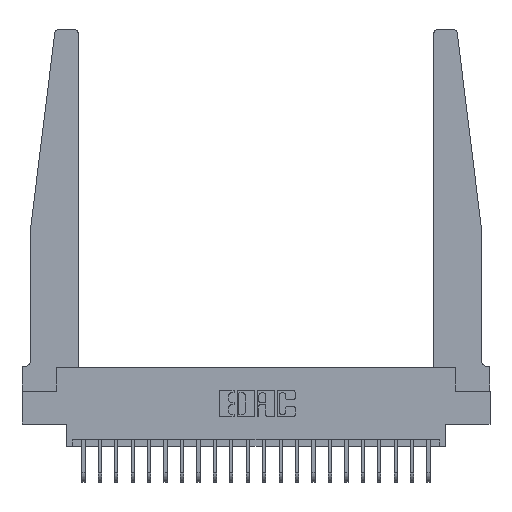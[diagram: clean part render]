
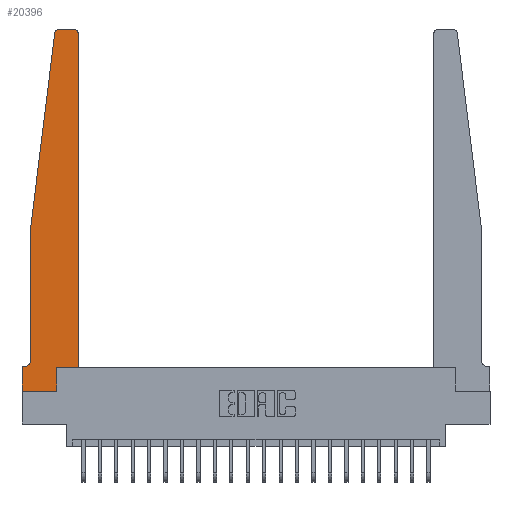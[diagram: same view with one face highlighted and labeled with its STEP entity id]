
A CAD part, top view. The second image highlights one B-rep face of the part: STEP entity #20396.
In plain terms, the highlighted planar face has unit normal (0, 0, 1).
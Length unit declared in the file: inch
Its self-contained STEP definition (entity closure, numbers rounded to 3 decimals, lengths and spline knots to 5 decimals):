
#13 = VERTEX_POINT ( 'NONE', #19878 ) ;
#154 = EDGE_CURVE ( 'NONE', #13275, #3862, #9523, .T. ) ;
#205 = VERTEX_POINT ( 'NONE', #922 ) ;
#274 = FACE_OUTER_BOUND ( 'NONE', #7038, .T. ) ;
#571 = CARTESIAN_POINT ( 'NONE',  ( 0., 0.1875, 0.37 ) ) ;
#922 = CARTESIAN_POINT ( 'NONE',  ( 0., 0., 0.37 ) ) ;
#1154 = EDGE_CURVE ( 'NONE', #13, #10740, #17629, .T. ) ;
#1171 = VECTOR ( 'NONE', #15582, 39.37008 ) ;
#1289 = CARTESIAN_POINT ( 'NONE',  ( 0., 0.1875, 0.37 ) ) ;
#2060 = VERTEX_POINT ( 'NONE', #20633 ) ;
#2206 = DIRECTION ( 'NONE',  ( 0., -1., 0. ) ) ;
#2225 = EDGE_CURVE ( 'NONE', #18120, #14885, #20172, .T. ) ;
#2480 = CARTESIAN_POINT ( 'NONE',  ( 0.2605, 0.18, 0.37 ) ) ;
#2614 = VECTOR ( 'NONE', #15246, 39.37008 ) ;
#2959 = DIRECTION ( 'NONE',  ( 1., 0., 0. ) ) ;
#3047 = LINE ( 'NONE', #4867, #7074 ) ;
#3566 = AXIS2_PLACEMENT_3D ( 'NONE', #14869, #5004, #16492 ) ;
#3673 = CARTESIAN_POINT ( 'NONE',  ( 0.395, 2.72, 0.37 ) ) ;
#3862 = VERTEX_POINT ( 'NONE', #5799 ) ;
#4046 = CIRCLE ( 'NONE', #3566, 0.03 ) ;
#4161 = CARTESIAN_POINT ( 'NONE',  ( 0.065, 1.25, 0.37 ) ) ;
#4199 = CARTESIAN_POINT ( 'NONE',  ( 0.425, 0.18, 0.37 ) ) ;
#4451 = ORIENTED_EDGE ( 'NONE', *, *, #12958, .T. ) ;
#4606 = CIRCLE ( 'NONE', #12302, 0.05 ) ;
#4867 = CARTESIAN_POINT ( 'NONE',  ( 0.425, 0.18, 0.37 ) ) ;
#4990 = ORIENTED_EDGE ( 'NONE', *, *, #1154, .T. ) ;
#5004 = DIRECTION ( 'NONE',  ( 0., 0., 1. ) ) ;
#5237 = ORIENTED_EDGE ( 'NONE', *, *, #8057, .T. ) ;
#5434 = DIRECTION ( 'NONE',  ( 1., 0., 0. ) ) ;
#5516 = ORIENTED_EDGE ( 'NONE', *, *, #20247, .T. ) ;
#5532 = EDGE_CURVE ( 'NONE', #12463, #2060, #11988, .T. ) ;
#5782 = CARTESIAN_POINT ( 'NONE',  ( 0., 0., 0.37 ) ) ;
#5799 = CARTESIAN_POINT ( 'NONE',  ( 0.065, 1.25, 0.37 ) ) ;
#6256 = VECTOR ( 'NONE', #2206, 39.37008 ) ;
#6421 = EDGE_CURVE ( 'NONE', #2060, #12313, #3047, .T. ) ;
#6766 = DIRECTION ( 'NONE',  ( 0., 0., -1. ) ) ;
#6806 = CARTESIAN_POINT ( 'NONE',  ( 0.25, 2.75, 0.37 ) ) ;
#7019 = CARTESIAN_POINT ( 'NONE',  ( 0.065, 0.1875, 0.37 ) ) ;
#7038 = EDGE_LOOP ( 'NONE', ( #4990, #4451, #19062, #10424, #18548, #14259, #5516, #13218, #8338, #16521, #14012, #5237 ) ) ;
#7074 = VECTOR ( 'NONE', #17970, 39.37008 ) ;
#7398 = VECTOR ( 'NONE', #10972, 39.37008 ) ;
#7460 = EDGE_CURVE ( 'NONE', #3862, #13134, #19252, .T. ) ;
#7509 = EDGE_CURVE ( 'NONE', #205, #12463, #18748, .T. ) ;
#7673 = CARTESIAN_POINT ( 'NONE',  ( 0., 0., 0.37 ) ) ;
#7940 = CARTESIAN_POINT ( 'NONE',  ( 0.27653, 2.75, 0.37 ) ) ;
#8057 = EDGE_CURVE ( 'NONE', #20066, #13, #17496, .T. ) ;
#8255 = CARTESIAN_POINT ( 'NONE',  ( 0.425, 0.18, 0.37 ) ) ;
#8338 = ORIENTED_EDGE ( 'NONE', *, *, #5532, .T. ) ;
#8434 = DIRECTION ( 'NONE',  ( -1., 0., 0. ) ) ;
#8803 = VECTOR ( 'NONE', #13204, 39.37008 ) ;
#9523 = LINE ( 'NONE', #4161, #17178 ) ;
#9659 = PLANE ( 'NONE',  #12207 ) ;
#10424 = ORIENTED_EDGE ( 'NONE', *, *, #7460, .T. ) ;
#10740 = VERTEX_POINT ( 'NONE', #7940 ) ;
#10853 = DIRECTION ( 'NONE',  ( 0., 1., 0. ) ) ;
#10972 = DIRECTION ( 'NONE',  ( 0., -1., 0. ) ) ;
#11455 = EDGE_CURVE ( 'NONE', #12313, #20066, #13160, .T. ) ;
#11749 = LINE ( 'NONE', #7673, #7398 ) ;
#11988 = LINE ( 'NONE', #2480, #19092 ) ;
#12207 = AXIS2_PLACEMENT_3D ( 'NONE', #1289, #12953, #2959 ) ;
#12302 = AXIS2_PLACEMENT_3D ( 'NONE', #16537, #6766, #18155 ) ;
#12313 = VERTEX_POINT ( 'NONE', #4199 ) ;
#12463 = VERTEX_POINT ( 'NONE', #19267 ) ;
#12953 = DIRECTION ( 'NONE',  ( 0., 0., 1. ) ) ;
#12958 = EDGE_CURVE ( 'NONE', #10740, #13275, #4046, .T. ) ;
#13134 = VERTEX_POINT ( 'NONE', #16837 ) ;
#13160 = LINE ( 'NONE', #8255, #8803 ) ;
#13204 = DIRECTION ( 'NONE',  ( 0., 1., 0. ) ) ;
#13218 = ORIENTED_EDGE ( 'NONE', *, *, #7509, .T. ) ;
#13275 = VERTEX_POINT ( 'NONE', #18811 ) ;
#13870 = CARTESIAN_POINT ( 'NONE',  ( 0.065, 1.25, 0.37 ) ) ;
#14012 = ORIENTED_EDGE ( 'NONE', *, *, #11455, .T. ) ;
#14259 = ORIENTED_EDGE ( 'NONE', *, *, #2225, .T. ) ;
#14869 = CARTESIAN_POINT ( 'NONE',  ( 0.27653, 2.72, 0.37 ) ) ;
#14885 = VERTEX_POINT ( 'NONE', #571 ) ;
#14989 = AXIS2_PLACEMENT_3D ( 'NONE', #3673, #15273, #5434 ) ;
#15246 = DIRECTION ( 'NONE',  ( -1., 0., 0. ) ) ;
#15273 = DIRECTION ( 'NONE',  ( 0., 0., 1. ) ) ;
#15582 = DIRECTION ( 'NONE',  ( 1., 0., 0. ) ) ;
#15711 = DIRECTION ( 'NONE',  ( -0.122, -0.992, 0. ) ) ;
#16492 = DIRECTION ( 'NONE',  ( 1., 0., 0. ) ) ;
#16521 = ORIENTED_EDGE ( 'NONE', *, *, #6421, .T. ) ;
#16537 = CARTESIAN_POINT ( 'NONE',  ( 0.015, 0.2375, 0.37 ) ) ;
#16837 = CARTESIAN_POINT ( 'NONE',  ( 0.065, 0.2375, 0.37 ) ) ;
#17178 = VECTOR ( 'NONE', #15711, 39.37008 ) ;
#17496 = CIRCLE ( 'NONE', #14989, 0.03 ) ;
#17629 = LINE ( 'NONE', #6806, #18644 ) ;
#17731 = EDGE_CURVE ( 'NONE', #13134, #18120, #4606, .T. ) ;
#17970 = DIRECTION ( 'NONE',  ( 1., 0., 0. ) ) ;
#18120 = VERTEX_POINT ( 'NONE', #20639 ) ;
#18155 = DIRECTION ( 'NONE',  ( -1., 0., 0. ) ) ;
#18548 = ORIENTED_EDGE ( 'NONE', *, *, #17731, .T. ) ;
#18644 = VECTOR ( 'NONE', #8434, 39.37008 ) ;
#18748 = LINE ( 'NONE', #5782, #1171 ) ;
#18811 = CARTESIAN_POINT ( 'NONE',  ( 0.24675, 2.72367, 0.37 ) ) ;
#19062 = ORIENTED_EDGE ( 'NONE', *, *, #154, .T. ) ;
#19092 = VECTOR ( 'NONE', #10853, 39.37008 ) ;
#19252 = LINE ( 'NONE', #13870, #6256 ) ;
#19267 = CARTESIAN_POINT ( 'NONE',  ( 0.2605, 0., 0.37 ) ) ;
#19878 = CARTESIAN_POINT ( 'NONE',  ( 0.395, 2.75, 0.37 ) ) ;
#20066 = VERTEX_POINT ( 'NONE', #20283 ) ;
#20172 = LINE ( 'NONE', #7019, #2614 ) ;
#20247 = EDGE_CURVE ( 'NONE', #14885, #205, #11749, .T. ) ;
#20283 = CARTESIAN_POINT ( 'NONE',  ( 0.425, 2.72, 0.37 ) ) ;
#20396 = ADVANCED_FACE ( 'NONE', ( #274 ), #9659, .T. ) ;
#20633 = CARTESIAN_POINT ( 'NONE',  ( 0.2605, 0.18, 0.37 ) ) ;
#20639 = CARTESIAN_POINT ( 'NONE',  ( 0.015, 0.1875, 0.37 ) ) ;
